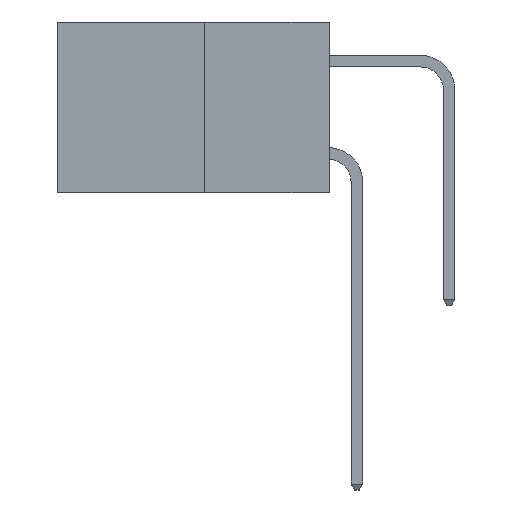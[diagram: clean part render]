
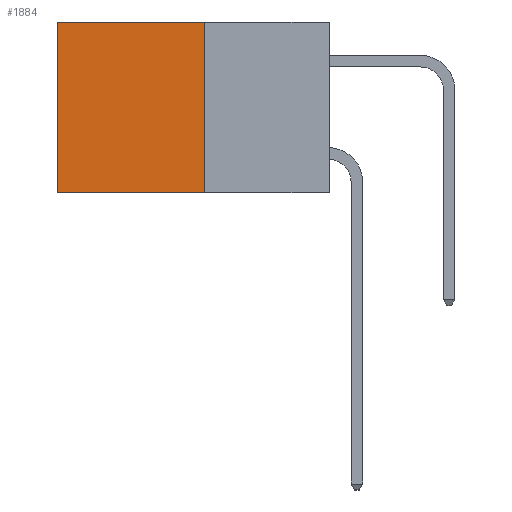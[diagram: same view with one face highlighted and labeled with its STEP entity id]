
A CAD part, left-side view. The second image highlights one B-rep face of the part: STEP entity #1884.
In plain terms, the highlighted planar face has unit normal (-1, 0, 0).
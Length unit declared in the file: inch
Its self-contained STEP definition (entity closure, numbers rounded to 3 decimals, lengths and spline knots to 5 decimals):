
#444 = EDGE_CURVE ( 'NONE', #9038, #4307, #9305, .T. ) ;
#1158 = DIRECTION ( 'NONE',  ( 0., 0., -1. ) ) ;
#1242 = DIRECTION ( 'NONE',  ( 1., 0., 0. ) ) ;
#1305 = VERTEX_POINT ( 'NONE', #8587 ) ;
#1411 = CARTESIAN_POINT ( 'NONE',  ( 0.277, 0.27, -0.37 ) ) ;
#1449 = LINE ( 'NONE', #4182, #12946 ) ;
#1457 = PLANE ( 'NONE',  #12672 ) ;
#1612 = VERTEX_POINT ( 'NONE', #11058 ) ;
#1884 = ADVANCED_FACE ( 'NONE', ( #19488 ), #1457, .F. ) ;
#2119 = ORIENTED_EDGE ( 'NONE', *, *, #15327, .F. ) ;
#2348 = EDGE_LOOP ( 'NONE', ( #15263, #2119, #18460, #16754 ) ) ;
#4182 = CARTESIAN_POINT ( 'NONE',  ( 0.277, 0.27, 0. ) ) ;
#4307 = VERTEX_POINT ( 'NONE', #7735 ) ;
#4507 = VECTOR ( 'NONE', #13313, 39.37008 ) ;
#4725 = EDGE_CURVE ( 'NONE', #1612, #1305, #5352, .T. ) ;
#4980 = LINE ( 'NONE', #5788, #4507 ) ;
#5224 = DIRECTION ( 'NONE',  ( 0., 0., -1. ) ) ;
#5352 = LINE ( 'NONE', #19304, #16433 ) ;
#5788 = CARTESIAN_POINT ( 'NONE',  ( 0.277, 0.27, -0.37 ) ) ;
#7735 = CARTESIAN_POINT ( 'NONE',  ( 0.277, 0.59, -0.37 ) ) ;
#7895 = CARTESIAN_POINT ( 'NONE',  ( 0.277, 0.59, 0. ) ) ;
#8587 = CARTESIAN_POINT ( 'NONE',  ( 0.277, 0.27, -0.37 ) ) ;
#8843 = VECTOR ( 'NONE', #5224, 39.37008 ) ;
#9038 = VERTEX_POINT ( 'NONE', #7895 ) ;
#9305 = LINE ( 'NONE', #19153, #8843 ) ;
#11058 = CARTESIAN_POINT ( 'NONE',  ( 0.277, 0.27, 0. ) ) ;
#11683 = DIRECTION ( 'NONE',  ( 0., 1., 0. ) ) ;
#12672 = AXIS2_PLACEMENT_3D ( 'NONE', #1411, #1242, #1158 ) ;
#12946 = VECTOR ( 'NONE', #11683, 39.37008 ) ;
#13313 = DIRECTION ( 'NONE',  ( 0., 1., 0. ) ) ;
#15263 = ORIENTED_EDGE ( 'NONE', *, *, #444, .T. ) ;
#15272 = EDGE_CURVE ( 'NONE', #1612, #9038, #1449, .T. ) ;
#15327 = EDGE_CURVE ( 'NONE', #1305, #4307, #4980, .T. ) ;
#16433 = VECTOR ( 'NONE', #19241, 39.37008 ) ;
#16754 = ORIENTED_EDGE ( 'NONE', *, *, #15272, .T. ) ;
#18460 = ORIENTED_EDGE ( 'NONE', *, *, #4725, .F. ) ;
#19153 = CARTESIAN_POINT ( 'NONE',  ( 0.277, 0.59, -0.37 ) ) ;
#19241 = DIRECTION ( 'NONE',  ( 0., 0., -1. ) ) ;
#19304 = CARTESIAN_POINT ( 'NONE',  ( 0.277, 0.27, -0.37 ) ) ;
#19488 = FACE_OUTER_BOUND ( 'NONE', #2348, .T. ) ;
